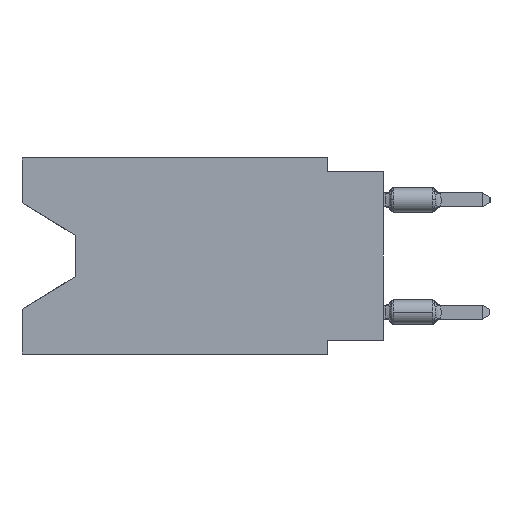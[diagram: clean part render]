
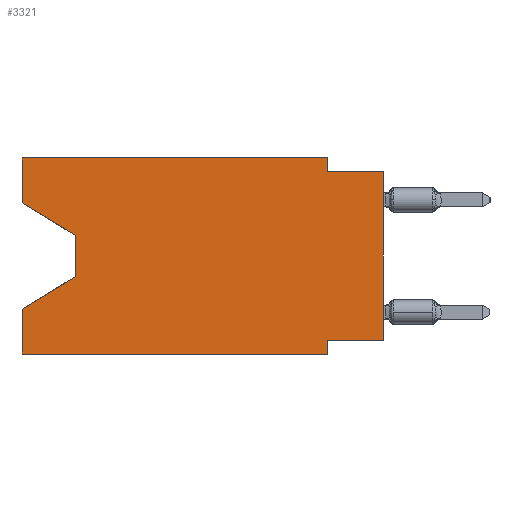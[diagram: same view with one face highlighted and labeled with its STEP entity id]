
A CAD part, left-side view. The second image highlights one B-rep face of the part: STEP entity #3321.
In plain terms, the highlighted planar face has unit normal (-1, 0, 0).
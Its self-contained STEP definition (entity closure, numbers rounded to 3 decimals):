
#907 = DIRECTION ( 'NONE',  ( 0., 0., -1. ) ) ;
#1456 = VERTEX_POINT ( 'NONE', #28382 ) ;
#1975 = VERTEX_POINT ( 'NONE', #3671 ) ;
#2202 = CARTESIAN_POINT ( 'NONE',  ( 0., 16.383, -2.038 ) ) ;
#2824 = VERTEX_POINT ( 'NONE', #15492 ) ;
#2905 = EDGE_CURVE ( 'NONE', #8769, #2824, #9125, .T. ) ;
#3321 = ADVANCED_FACE ( 'NONE', ( #26088 ), #34756, .F. ) ;
#3473 = ORIENTED_EDGE ( 'NONE', *, *, #32825, .F. ) ;
#3476 = CARTESIAN_POINT ( 'NONE',  ( 0., 16.383, 0. ) ) ;
#3671 = CARTESIAN_POINT ( 'NONE',  ( 0., 2.54, 0. ) ) ;
#3821 = DIRECTION ( 'NONE',  ( 0., -1., 0. ) ) ;
#3859 = CARTESIAN_POINT ( 'NONE',  ( 0., 16.383, 0. ) ) ;
#4390 = EDGE_CURVE ( 'NONE', #35780, #36144, #9972, .T. ) ;
#5005 = CARTESIAN_POINT ( 'NONE',  ( 0., 13.97, -5.385 ) ) ;
#5186 = VECTOR ( 'NONE', #19596, 1000. ) ;
#5188 = VECTOR ( 'NONE', #31291, 1000. ) ;
#5511 = ORIENTED_EDGE ( 'NONE', *, *, #2905, .T. ) ;
#5926 = CARTESIAN_POINT ( 'NONE',  ( 0., 2.54, 0. ) ) ;
#6044 = LINE ( 'NONE', #6385, #6995 ) ;
#6385 = CARTESIAN_POINT ( 'NONE',  ( 0., 16.383, 0. ) ) ;
#6426 = CARTESIAN_POINT ( 'NONE',  ( 0., 0., -0.635 ) ) ;
#6666 = ORIENTED_EDGE ( 'NONE', *, *, #35636, .T. ) ;
#6959 = VERTEX_POINT ( 'NONE', #12993 ) ;
#6995 = VECTOR ( 'NONE', #34468, 1000. ) ;
#7509 = VERTEX_POINT ( 'NONE', #26732 ) ;
#8079 = DIRECTION ( 'NONE',  ( 0., 0., 1. ) ) ;
#8466 = LINE ( 'NONE', #19878, #5188 ) ;
#8769 = VERTEX_POINT ( 'NONE', #20030 ) ;
#9125 = LINE ( 'NONE', #5005, #25092 ) ;
#9224 = ORIENTED_EDGE ( 'NONE', *, *, #25806, .F. ) ;
#9814 = LINE ( 'NONE', #3859, #17908 ) ;
#9901 = ORIENTED_EDGE ( 'NONE', *, *, #16288, .F. ) ;
#9972 = LINE ( 'NONE', #13184, #31764 ) ;
#10486 = ORIENTED_EDGE ( 'NONE', *, *, #4390, .F. ) ;
#10527 = DIRECTION ( 'NONE',  ( 0., 0., -1. ) ) ;
#11391 = ORIENTED_EDGE ( 'NONE', *, *, #27515, .T. ) ;
#12037 = VERTEX_POINT ( 'NONE', #26479 ) ;
#12380 = EDGE_CURVE ( 'NONE', #29112, #6959, #13725, .T. ) ;
#12657 = CARTESIAN_POINT ( 'NONE',  ( 0., 13.97, -3.505 ) ) ;
#12690 = LINE ( 'NONE', #21274, #25043 ) ;
#12993 = CARTESIAN_POINT ( 'NONE',  ( 0., 2.54, -8.89 ) ) ;
#13042 = EDGE_CURVE ( 'NONE', #1975, #12037, #31541, .T. ) ;
#13184 = CARTESIAN_POINT ( 'NONE',  ( 0., 0., -8.255 ) ) ;
#13725 = LINE ( 'NONE', #31128, #28623 ) ;
#14260 = CARTESIAN_POINT ( 'NONE',  ( 0., 0., -8.255 ) ) ;
#15049 = ORIENTED_EDGE ( 'NONE', *, *, #12380, .T. ) ;
#15259 = DIRECTION ( 'NONE',  ( 0., 0., 1. ) ) ;
#15492 = CARTESIAN_POINT ( 'NONE',  ( 0., 16.383, -6.852 ) ) ;
#16288 = EDGE_CURVE ( 'NONE', #36144, #6959, #12690, .T. ) ;
#16417 = LINE ( 'NONE', #2202, #5186 ) ;
#16906 = DIRECTION ( 'NONE',  ( 0., -1., 0. ) ) ;
#17168 = VECTOR ( 'NONE', #3821, 1000. ) ;
#17332 = DIRECTION ( 'NONE',  ( 0., 0., -1. ) ) ;
#17908 = VECTOR ( 'NONE', #15259, 1000. ) ;
#18576 = CARTESIAN_POINT ( 'NONE',  ( 0., 16.383, 0. ) ) ;
#19170 = VERTEX_POINT ( 'NONE', #12657 ) ;
#19596 = DIRECTION ( 'NONE',  ( 0., -0.855, -0.519 ) ) ;
#19631 = VECTOR ( 'NONE', #8079, 1000. ) ;
#19692 = CARTESIAN_POINT ( 'NONE',  ( 0., 0., 0. ) ) ;
#19878 = CARTESIAN_POINT ( 'NONE',  ( 0., 16.383, 0. ) ) ;
#20030 = CARTESIAN_POINT ( 'NONE',  ( 0., 13.97, -5.385 ) ) ;
#20465 = LINE ( 'NONE', #6426, #17168 ) ;
#20806 = EDGE_CURVE ( 'NONE', #12037, #1456, #20465, .T. ) ;
#21274 = CARTESIAN_POINT ( 'NONE',  ( 0., 2.54, -8.89 ) ) ;
#21822 = CARTESIAN_POINT ( 'NONE',  ( 0., 16.383, -8.89 ) ) ;
#22007 = DIRECTION ( 'NONE',  ( 0., 0.855, -0.519 ) ) ;
#25043 = VECTOR ( 'NONE', #907, 1000. ) ;
#25092 = VECTOR ( 'NONE', #22007, 1000. ) ;
#25806 = EDGE_CURVE ( 'NONE', #28070, #1975, #8466, .T. ) ;
#26088 = FACE_OUTER_BOUND ( 'NONE', #26744, .T. ) ;
#26298 = DIRECTION ( 'NONE',  ( 1., 0., 0. ) ) ;
#26479 = CARTESIAN_POINT ( 'NONE',  ( 0., 2.54, -0.635 ) ) ;
#26732 = CARTESIAN_POINT ( 'NONE',  ( 0., 16.383, -2.038 ) ) ;
#26744 = EDGE_LOOP ( 'NONE', ( #11391, #35615, #5511, #3473, #15049, #9901, #10486, #6666, #29012, #36186, #9224, #31808 ) ) ;
#27515 = EDGE_CURVE ( 'NONE', #7509, #19170, #16417, .T. ) ;
#28070 = VERTEX_POINT ( 'NONE', #18576 ) ;
#28382 = CARTESIAN_POINT ( 'NONE',  ( 0., 0., -0.635 ) ) ;
#28623 = VECTOR ( 'NONE', #16906, 1000. ) ;
#28947 = EDGE_CURVE ( 'NONE', #19170, #8769, #32521, .T. ) ;
#29012 = ORIENTED_EDGE ( 'NONE', *, *, #20806, .F. ) ;
#29099 = VECTOR ( 'NONE', #17332, 1000. ) ;
#29112 = VERTEX_POINT ( 'NONE', #21822 ) ;
#30634 = EDGE_CURVE ( 'NONE', #7509, #28070, #9814, .T. ) ;
#31128 = CARTESIAN_POINT ( 'NONE',  ( 0., 16.383, -8.89 ) ) ;
#31291 = DIRECTION ( 'NONE',  ( 0., -1., 0. ) ) ;
#31541 = LINE ( 'NONE', #5926, #29099 ) ;
#31764 = VECTOR ( 'NONE', #33025, 1000. ) ;
#31808 = ORIENTED_EDGE ( 'NONE', *, *, #30634, .F. ) ;
#32521 = LINE ( 'NONE', #32899, #33346 ) ;
#32825 = EDGE_CURVE ( 'NONE', #29112, #2824, #6044, .T. ) ;
#32899 = CARTESIAN_POINT ( 'NONE',  ( 0., 13.97, -3.505 ) ) ;
#33025 = DIRECTION ( 'NONE',  ( 0., 1., 0. ) ) ;
#33346 = VECTOR ( 'NONE', #35171, 1000. ) ;
#34077 = CARTESIAN_POINT ( 'NONE',  ( 0., 2.54, -8.255 ) ) ;
#34468 = DIRECTION ( 'NONE',  ( 0., 0., 1. ) ) ;
#34756 = PLANE ( 'NONE',  #36524 ) ;
#35171 = DIRECTION ( 'NONE',  ( 0., 0., -1. ) ) ;
#35615 = ORIENTED_EDGE ( 'NONE', *, *, #28947, .T. ) ;
#35636 = EDGE_CURVE ( 'NONE', #35780, #1456, #36034, .T. ) ;
#35780 = VERTEX_POINT ( 'NONE', #14260 ) ;
#36034 = LINE ( 'NONE', #19692, #19631 ) ;
#36144 = VERTEX_POINT ( 'NONE', #34077 ) ;
#36186 = ORIENTED_EDGE ( 'NONE', *, *, #13042, .F. ) ;
#36524 = AXIS2_PLACEMENT_3D ( 'NONE', #3476, #26298, #10527 ) ;
